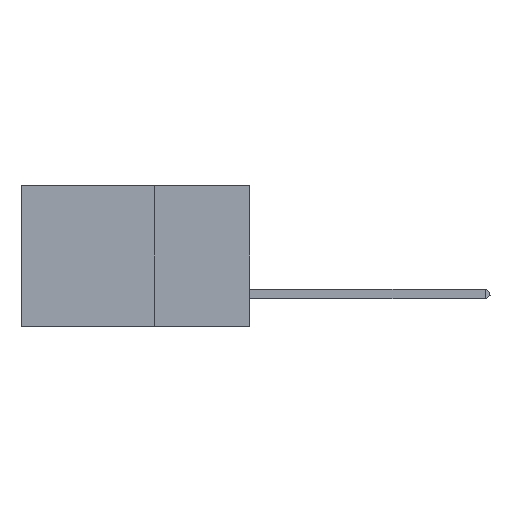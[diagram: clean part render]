
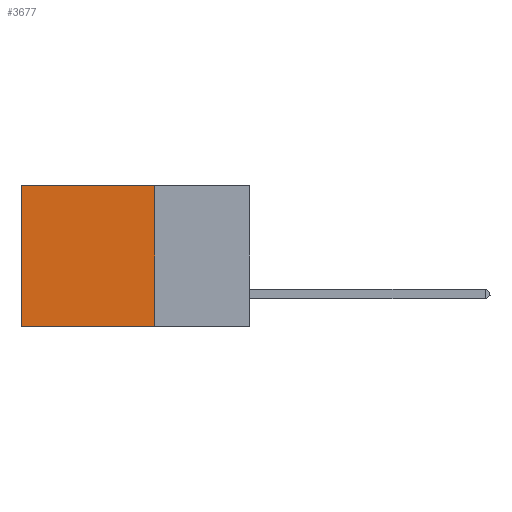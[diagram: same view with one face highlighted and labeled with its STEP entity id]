
A CAD part, left-side view. The second image highlights one B-rep face of the part: STEP entity #3677.
In plain terms, the highlighted planar face has unit normal (-1, 0, 0).
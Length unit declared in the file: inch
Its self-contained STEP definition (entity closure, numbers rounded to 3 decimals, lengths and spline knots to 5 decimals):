
#414 = VECTOR ( 'NONE', #3447, 39.37008 ) ;
#1673 = CARTESIAN_POINT ( 'NONE',  ( 0.2875, 0.25, -0.37 ) ) ;
#1803 = PLANE ( 'NONE',  #8956 ) ;
#1844 = CARTESIAN_POINT ( 'NONE',  ( 0.2875, 0.6, 0. ) ) ;
#2098 = ORIENTED_EDGE ( 'NONE', *, *, #13854, .T. ) ;
#2475 = EDGE_CURVE ( 'NONE', #16051, #8544, #12836, .T. ) ;
#2514 = VECTOR ( 'NONE', #9794, 39.37008 ) ;
#2536 = CARTESIAN_POINT ( 'NONE',  ( 0.2875, 0.25, 0. ) ) ;
#3447 = DIRECTION ( 'NONE',  ( 0., 0., -1. ) ) ;
#3677 = ADVANCED_FACE ( 'NONE', ( #14854 ), #1803, .F. ) ;
#3826 = VERTEX_POINT ( 'NONE', #1844 ) ;
#5357 = CARTESIAN_POINT ( 'NONE',  ( 0.2875, 0.6, -0.37 ) ) ;
#7731 = ORIENTED_EDGE ( 'NONE', *, *, #16771, .F. ) ;
#7978 = LINE ( 'NONE', #19509, #414 ) ;
#8544 = VERTEX_POINT ( 'NONE', #5357 ) ;
#8956 = AXIS2_PLACEMENT_3D ( 'NONE', #12844, #11317, #16269 ) ;
#9093 = ORIENTED_EDGE ( 'NONE', *, *, #2475, .F. ) ;
#9794 = DIRECTION ( 'NONE',  ( 0., 0., -1. ) ) ;
#9881 = VECTOR ( 'NONE', #15411, 39.37008 ) ;
#10417 = VERTEX_POINT ( 'NONE', #2536 ) ;
#10607 = VECTOR ( 'NONE', #17381, 39.37008 ) ;
#11118 = LINE ( 'NONE', #18608, #9881 ) ;
#11317 = DIRECTION ( 'NONE',  ( 1., 0., 0. ) ) ;
#12006 = EDGE_LOOP ( 'NONE', ( #2098, #9093, #7731, #12471 ) ) ;
#12471 = ORIENTED_EDGE ( 'NONE', *, *, #18289, .T. ) ;
#12836 = LINE ( 'NONE', #1673, #10607 ) ;
#12844 = CARTESIAN_POINT ( 'NONE',  ( 0.2875, 0.25, 0. ) ) ;
#13854 = EDGE_CURVE ( 'NONE', #3826, #8544, #7978, .T. ) ;
#14854 = FACE_OUTER_BOUND ( 'NONE', #12006, .T. ) ;
#15411 = DIRECTION ( 'NONE',  ( 0., 1., 0. ) ) ;
#16051 = VERTEX_POINT ( 'NONE', #18907 ) ;
#16269 = DIRECTION ( 'NONE',  ( 0., 0., -1. ) ) ;
#16771 = EDGE_CURVE ( 'NONE', #10417, #16051, #20055, .T. ) ;
#17381 = DIRECTION ( 'NONE',  ( 0., 1., 0. ) ) ;
#18289 = EDGE_CURVE ( 'NONE', #10417, #3826, #11118, .T. ) ;
#18608 = CARTESIAN_POINT ( 'NONE',  ( 0.2875, 0.25, 0. ) ) ;
#18907 = CARTESIAN_POINT ( 'NONE',  ( 0.2875, 0.25, -0.37 ) ) ;
#19316 = CARTESIAN_POINT ( 'NONE',  ( 0.2875, 0.25, 0. ) ) ;
#19509 = CARTESIAN_POINT ( 'NONE',  ( 0.2875, 0.6, 0. ) ) ;
#20055 = LINE ( 'NONE', #19316, #2514 ) ;
